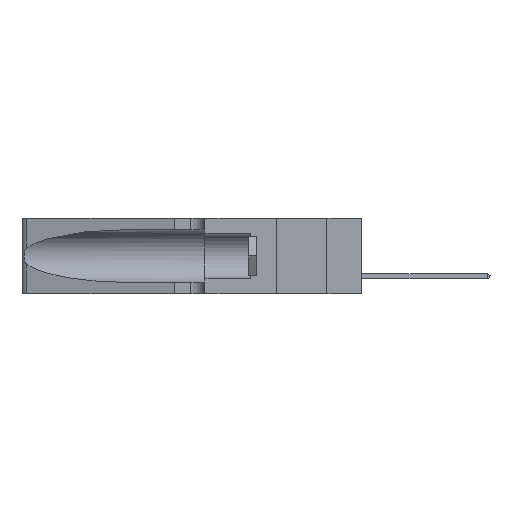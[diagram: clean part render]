
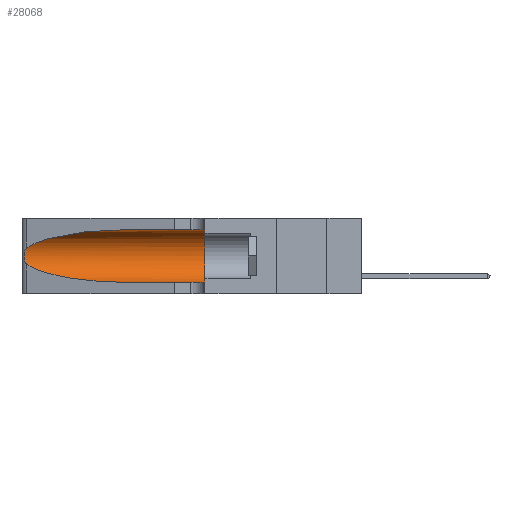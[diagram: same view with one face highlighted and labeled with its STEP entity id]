
A CAD part, left-side view. The second image highlights one B-rep face of the part: STEP entity #28068.
In plain terms, the highlighted cylindrical face has radius 3.308 mm (diameter 6.617 mm), a partial arc.
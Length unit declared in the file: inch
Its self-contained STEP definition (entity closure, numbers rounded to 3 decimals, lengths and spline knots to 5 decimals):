
#116 = CARTESIAN_POINT ( 'NONE',  ( 0.1305, 1.61858, 0.185 ) ) ;
#196 = CARTESIAN_POINT ( 'NONE',  ( 0.25487, 1.22718, 0.14631 ) ) ;
#935 = VECTOR ( 'NONE', #41194, 39.37008 ) ;
#1219 = EDGE_CURVE ( 'NONE', #1233, #40929, #9447, .T. ) ;
#1233 = VERTEX_POINT ( 'NONE', #23943 ) ;
#1260 = CARTESIAN_POINT ( 'NONE',  ( 0.1305, 0.72297, 0.05475 ) ) ;
#1451 = CARTESIAN_POINT ( 'NONE',  ( 0.1305, 0.72297, 0.31525 ) ) ;
#1799 = CARTESIAN_POINT ( 'NONE',  ( 0.2373, 1.15595, 0.08982 ) ) ;
#2424 = CARTESIAN_POINT ( 'NONE',  ( 0.1305, 0.72297, 0.31525 ) ) ;
#2932 = DIRECTION ( 'NONE',  ( 0., -1., 0. ) ) ;
#3986 = CARTESIAN_POINT ( 'NONE',  ( 0.25555, 1.22994, 0.2215 ) ) ;
#4037 =( BOUNDED_CURVE ( )  B_SPLINE_CURVE ( 3, ( #29052, #1799, #6059, #1260 ),
 .UNSPECIFIED., .F., .F. ) 
 B_SPLINE_CURVE_WITH_KNOTS ( ( 4, 4 ),
 ( 3.44316, 4.71239 ),
 .UNSPECIFIED. ) 
 CURVE ( )  GEOMETRIC_REPRESENTATION_ITEM ( )  RATIONAL_B_SPLINE_CURVE ( ( 1., 0.87, 0.87, 1. ) ) 
 REPRESENTATION_ITEM ( '' )  );
#5741 = CARTESIAN_POINT ( 'NONE',  ( 0.25487, 1.22718, 0.22369 ) ) ;
#5894 = CARTESIAN_POINT ( 'NONE',  ( 0.25639, 1.23184, 0.21858 ) ) ;
#5903 = VERTEX_POINT ( 'NONE', #1451 ) ;
#6059 = CARTESIAN_POINT ( 'NONE',  ( 0.18966, 0.96281, 0.05475 ) ) ;
#6299 = EDGE_CURVE ( 'NONE', #39936, #1233, #4037, .T. ) ;
#6333 = ORIENTED_EDGE ( 'NONE', *, *, #1219, .T. ) ;
#6399 = VERTEX_POINT ( 'NONE', #30613 ) ;
#6470 = DIRECTION ( 'NONE',  ( 0., -1., 0. ) ) ;
#6711 = AXIS2_PLACEMENT_3D ( 'NONE', #21798, #11684, #38085 ) ;
#6741 = CARTESIAN_POINT ( 'NONE',  ( 0.25787, 1.23484, 0.2124 ) ) ;
#7007 = CARTESIAN_POINT ( 'NONE',  ( 0.25856, 1.23593, 0.16098 ) ) ;
#7043 = FACE_OUTER_BOUND ( 'NONE', #15074, .T. ) ;
#8770 = ORIENTED_EDGE ( 'NONE', *, *, #6299, .T. ) ;
#9447 = LINE ( 'NONE', #22110, #34470 ) ;
#11684 = DIRECTION ( 'NONE',  ( 0., 1., 0. ) ) ;
#12626 = CARTESIAN_POINT ( 'NONE',  ( 0.25487, 1.22718, 0.14631 ) ) ;
#13317 = CYLINDRICAL_SURFACE ( 'NONE', #42159, 0.13025 ) ;
#13468 = CARTESIAN_POINT ( 'NONE',  ( 0.25789, 1.23486, 0.15765 ) ) ;
#14485 =( BOUNDED_CURVE ( )  B_SPLINE_CURVE ( 3, ( #2424, #29219, #35624, #5741 ),
 .UNSPECIFIED., .F., .F. ) 
 B_SPLINE_CURVE_WITH_KNOTS ( ( 4, 4 ),
 ( 1.5708, 2.84003 ),
 .UNSPECIFIED. ) 
 CURVE ( )  GEOMETRIC_REPRESENTATION_ITEM ( )  RATIONAL_B_SPLINE_CURVE ( ( 1., 0.87, 0.87, 1. ) ) 
 REPRESENTATION_ITEM ( '' )  );
#15074 = EDGE_LOOP ( 'NONE', ( #25697, #20946, #8770, #6333, #21725, #29559 ) ) ;
#15114 = EDGE_CURVE ( 'NONE', #5903, #16490, #14485, .T. ) ;
#16161 = DIRECTION ( 'NONE',  ( 0., 0., -1. ) ) ;
#16490 = VERTEX_POINT ( 'NONE', #29527 ) ;
#16615 = EDGE_CURVE ( 'NONE', #6399, #40929, #22018, .T. ) ;
#17253 = CARTESIAN_POINT ( 'NONE',  ( 0.25487, 1.22718, 0.22369 ) ) ;
#20946 = ORIENTED_EDGE ( 'NONE', *, *, #32595, .T. ) ;
#21725 = ORIENTED_EDGE ( 'NONE', *, *, #16615, .F. ) ;
#21798 = CARTESIAN_POINT ( 'NONE',  ( 0.1305, 0.35, 0.185 ) ) ;
#22018 = CIRCLE ( 'NONE', #6711, 0.13025 ) ;
#22110 = CARTESIAN_POINT ( 'NONE',  ( 0.1305, 1.61858, 0.05475 ) ) ;
#23943 = CARTESIAN_POINT ( 'NONE',  ( 0.1305, 0.72297, 0.05475 ) ) ;
#25697 = ORIENTED_EDGE ( 'NONE', *, *, #15114, .T. ) ;
#25929 = CARTESIAN_POINT ( 'NONE',  ( 0.25854, 1.2359, 0.20912 ) ) ;
#27019 = CARTESIAN_POINT ( 'NONE',  ( 0.26075, 1.23896, 0.178 ) ) ;
#28068 = ADVANCED_FACE ( 'NONE', ( #7043 ), #13317, .F. ) ;
#29052 = CARTESIAN_POINT ( 'NONE',  ( 0.25487, 1.22718, 0.14631 ) ) ;
#29214 = CARTESIAN_POINT ( 'NONE',  ( 0.26018, 1.23835, 0.19895 ) ) ;
#29219 = CARTESIAN_POINT ( 'NONE',  ( 0.18966, 0.96281, 0.31525 ) ) ;
#29527 = CARTESIAN_POINT ( 'NONE',  ( 0.25487, 1.22718, 0.22369 ) ) ;
#29559 = ORIENTED_EDGE ( 'NONE', *, *, #32180, .F. ) ;
#30613 = CARTESIAN_POINT ( 'NONE',  ( 0.1305, 0.35, 0.31525 ) ) ;
#32180 = EDGE_CURVE ( 'NONE', #5903, #6399, #38510, .T. ) ;
#32595 = EDGE_CURVE ( 'NONE', #16490, #39936, #40942, .T. ) ;
#33299 = CARTESIAN_POINT ( 'NONE',  ( 0.26075, 1.23896, 0.19203 ) ) ;
#33416 = CARTESIAN_POINT ( 'NONE',  ( 0.26017, 1.23833, 0.17102 ) ) ;
#34470 = VECTOR ( 'NONE', #6470, 39.37008 ) ;
#35624 = CARTESIAN_POINT ( 'NONE',  ( 0.2373, 1.15595, 0.28018 ) ) ;
#36632 = CARTESIAN_POINT ( 'NONE',  ( 0.25555, 1.22993, 0.14849 ) ) ;
#38085 = DIRECTION ( 'NONE',  ( 0., 0., 1. ) ) ;
#38165 = CARTESIAN_POINT ( 'NONE',  ( 0.1305, 0.35, 0.05475 ) ) ;
#38510 = LINE ( 'NONE', #41793, #935 ) ;
#39936 = VERTEX_POINT ( 'NONE', #12626 ) ;
#40135 = CARTESIAN_POINT ( 'NONE',  ( 0.25639, 1.23186, 0.15144 ) ) ;
#40929 = VERTEX_POINT ( 'NONE', #38165 ) ;
#40942 = B_SPLINE_CURVE_WITH_KNOTS ( 'NONE', 3,
 ( #17253, #3986, #5894, #6741, #25929, #29214, #33299, #27019, #33416, #7007, #13468, #40135, #36632, #196 ),
 .UNSPECIFIED., .F., .F.,
 ( 4, 2, 2, 2, 2, 2, 4 ),
 ( 0., 0.00027, 0.00053, 0.00107, 0.0016, 0.00187, 0.00214 ),
 .UNSPECIFIED. ) ;
#41194 = DIRECTION ( 'NONE',  ( 0., -1., 0. ) ) ;
#41793 = CARTESIAN_POINT ( 'NONE',  ( 0.1305, 1.61858, 0.31525 ) ) ;
#42159 = AXIS2_PLACEMENT_3D ( 'NONE', #116, #2932, #16161 ) ;
